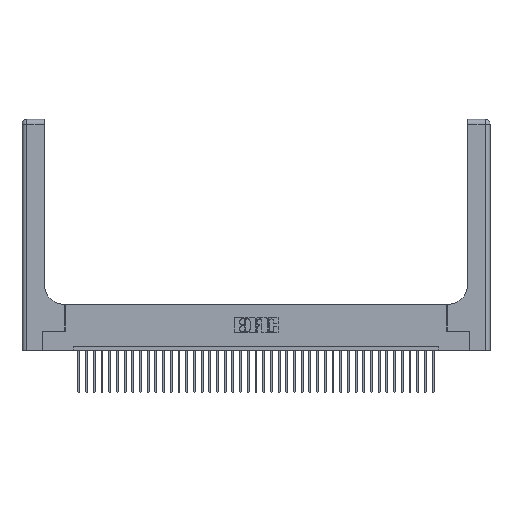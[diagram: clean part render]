
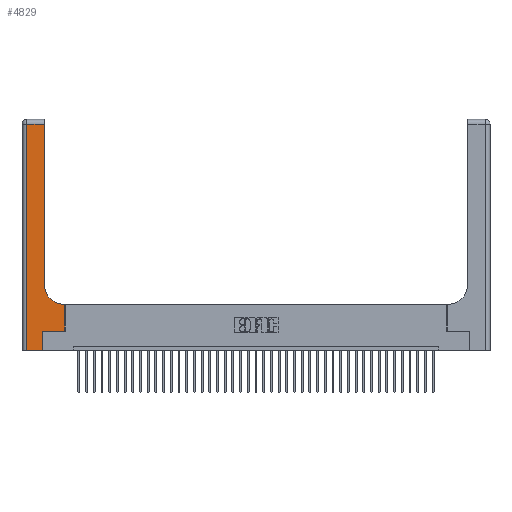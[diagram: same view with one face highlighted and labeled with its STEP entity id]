
A CAD part, top view. The second image highlights one B-rep face of the part: STEP entity #4829.
In plain terms, the highlighted planar face has unit normal (0, 0, 1).
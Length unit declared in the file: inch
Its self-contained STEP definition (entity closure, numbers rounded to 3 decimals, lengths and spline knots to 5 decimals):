
#157 = CARTESIAN_POINT ( 'NONE',  ( 0., 0., 0.37 ) ) ;
#523 = VECTOR ( 'NONE', #14898, 39.37008 ) ;
#1124 = LINE ( 'NONE', #33835, #27197 ) ;
#1160 = DIRECTION ( 'NONE',  ( 0., 1., 0. ) ) ;
#1276 = EDGE_CURVE ( 'NONE', #32530, #2844, #3908, .T. ) ;
#1679 = FACE_OUTER_BOUND ( 'NONE', #2054, .T. ) ;
#2054 = EDGE_LOOP ( 'NONE', ( #30311, #28841, #17200, #34485, #4432, #16099, #17465, #27018, #33899 ) ) ;
#2168 = EDGE_CURVE ( 'NONE', #13314, #30316, #20339, .T. ) ;
#2357 = VERTEX_POINT ( 'NONE', #9920 ) ;
#2844 = VERTEX_POINT ( 'NONE', #35128 ) ;
#2881 = LINE ( 'NONE', #28699, #6686 ) ;
#3908 = LINE ( 'NONE', #18024, #36721 ) ;
#4027 = VECTOR ( 'NONE', #19795, 39.37008 ) ;
#4032 = DIRECTION ( 'NONE',  ( -1., 0., 0. ) ) ;
#4222 = PLANE ( 'NONE',  #37116 ) ;
#4324 = VECTOR ( 'NONE', #30103, 39.37008 ) ;
#4432 = ORIENTED_EDGE ( 'NONE', *, *, #2168, .T. ) ;
#4829 = ADVANCED_FACE ( 'NONE', ( #1679 ), #4222, .F. ) ;
#5329 = EDGE_CURVE ( 'NONE', #2357, #32530, #1124, .T. ) ;
#5429 = CARTESIAN_POINT ( 'NONE',  ( 0.269, 0., 0.37 ) ) ;
#5625 = CARTESIAN_POINT ( 'NONE',  ( 0.06, 0., 0.37 ) ) ;
#6686 = VECTOR ( 'NONE', #22412, 39.37008 ) ;
#7814 = CARTESIAN_POINT ( 'NONE',  ( 0.269, 0.25, 0.37 ) ) ;
#8859 = AXIS2_PLACEMENT_3D ( 'NONE', #23775, #11326, #26971 ) ;
#8867 = VECTOR ( 'NONE', #1160, 39.37008 ) ;
#9920 = CARTESIAN_POINT ( 'NONE',  ( 0.2915, 0.85, 0.37 ) ) ;
#10014 = EDGE_CURVE ( 'NONE', #32412, #2357, #38228, .T. ) ;
#10864 = EDGE_CURVE ( 'NONE', #2844, #23143, #12575, .T. ) ;
#11326 = DIRECTION ( 'NONE',  ( 0., 0., -1. ) ) ;
#12064 = DIRECTION ( 'NONE',  ( 0., 1., 0. ) ) ;
#12575 = LINE ( 'NONE', #30014, #523 ) ;
#13271 = VERTEX_POINT ( 'NONE', #24280 ) ;
#13314 = VERTEX_POINT ( 'NONE', #33775 ) ;
#14681 = LINE ( 'NONE', #19687, #8867 ) ;
#14898 = DIRECTION ( 'NONE',  ( 0., -1., 0. ) ) ;
#14988 = CARTESIAN_POINT ( 'NONE',  ( 0., 3., 0.37 ) ) ;
#15561 = LINE ( 'NONE', #32130, #4027 ) ;
#15704 = CARTESIAN_POINT ( 'NONE',  ( 0.5585, 0.6, 0.37 ) ) ;
#16099 = ORIENTED_EDGE ( 'NONE', *, *, #38898, .T. ) ;
#17200 = ORIENTED_EDGE ( 'NONE', *, *, #10864, .T. ) ;
#17465 = ORIENTED_EDGE ( 'NONE', *, *, #23741, .T. ) ;
#18024 = CARTESIAN_POINT ( 'NONE',  ( 0., 2.94, 0.37 ) ) ;
#19635 = DIRECTION ( 'NONE',  ( 1., 0., 0. ) ) ;
#19687 = CARTESIAN_POINT ( 'NONE',  ( 0.5585, 0.25, 0.37 ) ) ;
#19795 = DIRECTION ( 'NONE',  ( 1., 0., 0. ) ) ;
#20339 = LINE ( 'NONE', #5429, #4324 ) ;
#21023 = VERTEX_POINT ( 'NONE', #15704 ) ;
#22412 = DIRECTION ( 'NONE',  ( -1., 0., 0. ) ) ;
#22633 = CARTESIAN_POINT ( 'NONE',  ( 0.5415, 0.6, 0.37 ) ) ;
#23143 = VERTEX_POINT ( 'NONE', #5625 ) ;
#23741 = EDGE_CURVE ( 'NONE', #13271, #21023, #14681, .T. ) ;
#23775 = CARTESIAN_POINT ( 'NONE',  ( 0.5415, 0.85, 0.37 ) ) ;
#24280 = CARTESIAN_POINT ( 'NONE',  ( 0.5585, 0.25, 0.37 ) ) ;
#25451 = LINE ( 'NONE', #157, #37010 ) ;
#26833 = EDGE_CURVE ( 'NONE', #23143, #13314, #25451, .T. ) ;
#26971 = DIRECTION ( 'NONE',  ( 1., 0., 0. ) ) ;
#27018 = ORIENTED_EDGE ( 'NONE', *, *, #36359, .T. ) ;
#27197 = VECTOR ( 'NONE', #12064, 39.37008 ) ;
#28699 = CARTESIAN_POINT ( 'NONE',  ( 0.2915, 0.6, 0.37 ) ) ;
#28841 = ORIENTED_EDGE ( 'NONE', *, *, #1276, .T. ) ;
#30014 = CARTESIAN_POINT ( 'NONE',  ( 0.06, 3., 0.37 ) ) ;
#30103 = DIRECTION ( 'NONE',  ( 0., 1., 0. ) ) ;
#30311 = ORIENTED_EDGE ( 'NONE', *, *, #5329, .T. ) ;
#30316 = VERTEX_POINT ( 'NONE', #7814 ) ;
#32130 = CARTESIAN_POINT ( 'NONE',  ( 0.269, 0.25, 0.37 ) ) ;
#32412 = VERTEX_POINT ( 'NONE', #22633 ) ;
#32530 = VERTEX_POINT ( 'NONE', #38343 ) ;
#33775 = CARTESIAN_POINT ( 'NONE',  ( 0.269, 0., 0.37 ) ) ;
#33835 = CARTESIAN_POINT ( 'NONE',  ( 0.2915, 3., 0.37 ) ) ;
#33855 = DIRECTION ( 'NONE',  ( -1., 0., 0. ) ) ;
#33899 = ORIENTED_EDGE ( 'NONE', *, *, #10014, .T. ) ;
#34485 = ORIENTED_EDGE ( 'NONE', *, *, #26833, .T. ) ;
#35128 = CARTESIAN_POINT ( 'NONE',  ( 0.06, 2.94, 0.37 ) ) ;
#36359 = EDGE_CURVE ( 'NONE', #21023, #32412, #2881, .T. ) ;
#36721 = VECTOR ( 'NONE', #33855, 39.37008 ) ;
#37010 = VECTOR ( 'NONE', #19635, 39.37008 ) ;
#37116 = AXIS2_PLACEMENT_3D ( 'NONE', #14988, #37269, #4032 ) ;
#37269 = DIRECTION ( 'NONE',  ( 0., 0., -1. ) ) ;
#38228 = CIRCLE ( 'NONE', #8859, 0.25 ) ;
#38343 = CARTESIAN_POINT ( 'NONE',  ( 0.2915, 2.94, 0.37 ) ) ;
#38898 = EDGE_CURVE ( 'NONE', #30316, #13271, #15561, .T. ) ;
